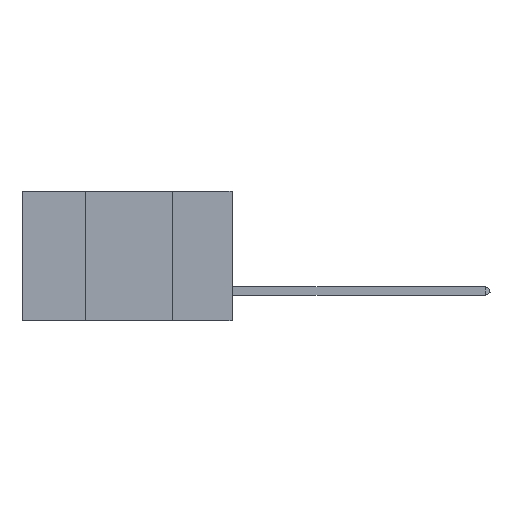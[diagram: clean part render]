
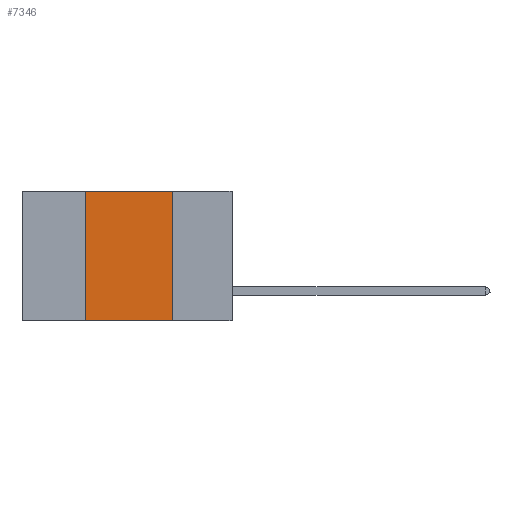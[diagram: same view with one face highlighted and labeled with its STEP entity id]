
A CAD part, left-side view. The second image highlights one B-rep face of the part: STEP entity #7346.
In plain terms, the highlighted planar face has unit normal (-1, 0, 0).
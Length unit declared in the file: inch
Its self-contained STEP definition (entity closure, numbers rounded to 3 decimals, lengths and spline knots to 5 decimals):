
#81 = CARTESIAN_POINT ( 'NONE',  ( 0., 0.6, 0. ) ) ;
#466 = CARTESIAN_POINT ( 'NONE',  ( 0., 0.17, 0. ) ) ;
#743 = EDGE_CURVE ( 'NONE', #13435, #10442, #17236, .T. ) ;
#807 = LINE ( 'NONE', #81, #6504 ) ;
#971 = CARTESIAN_POINT ( 'NONE',  ( 0., 0.6, -0.37 ) ) ;
#2218 = EDGE_LOOP ( 'NONE', ( #6266, #3308, #15476, #9253 ) ) ;
#3107 = LINE ( 'NONE', #971, #4818 ) ;
#3308 = ORIENTED_EDGE ( 'NONE', *, *, #3392, .F. ) ;
#3386 = DIRECTION ( 'NONE',  ( 0., 0., 1. ) ) ;
#3392 = EDGE_CURVE ( 'NONE', #9816, #13435, #807, .T. ) ;
#4089 = DIRECTION ( 'NONE',  ( 1., 0., 0. ) ) ;
#4458 = EDGE_CURVE ( 'NONE', #15866, #9816, #14461, .T. ) ;
#4818 = VECTOR ( 'NONE', #11678, 39.37008 ) ;
#5842 = CARTESIAN_POINT ( 'NONE',  ( 0., 0.17, -0.37 ) ) ;
#6266 = ORIENTED_EDGE ( 'NONE', *, *, #743, .F. ) ;
#6504 = VECTOR ( 'NONE', #17432, 39.37008 ) ;
#6873 = CARTESIAN_POINT ( 'NONE',  ( 0., 0.17, 0. ) ) ;
#6984 = CARTESIAN_POINT ( 'NONE',  ( 0., 0.42, -0.37 ) ) ;
#7245 = AXIS2_PLACEMENT_3D ( 'NONE', #13342, #4089, #10845 ) ;
#7313 = CARTESIAN_POINT ( 'NONE',  ( 0., 0.42, 0. ) ) ;
#7346 = ADVANCED_FACE ( 'NONE', ( #11368 ), #10675, .F. ) ;
#8486 = DIRECTION ( 'NONE',  ( 0., 0., -1. ) ) ;
#9253 = ORIENTED_EDGE ( 'NONE', *, *, #16838, .T. ) ;
#9453 = CARTESIAN_POINT ( 'NONE',  ( 0., 0.42, 0. ) ) ;
#9816 = VERTEX_POINT ( 'NONE', #9453 ) ;
#10442 = VERTEX_POINT ( 'NONE', #5842 ) ;
#10629 = VECTOR ( 'NONE', #3386, 39.37008 ) ;
#10675 = PLANE ( 'NONE',  #7245 ) ;
#10845 = DIRECTION ( 'NONE',  ( 0., 0., -1. ) ) ;
#11368 = FACE_OUTER_BOUND ( 'NONE', #2218, .T. ) ;
#11678 = DIRECTION ( 'NONE',  ( 0., -1., 0. ) ) ;
#13342 = CARTESIAN_POINT ( 'NONE',  ( 0., 0.6, 0. ) ) ;
#13435 = VERTEX_POINT ( 'NONE', #6873 ) ;
#14043 = VECTOR ( 'NONE', #8486, 39.37008 ) ;
#14461 = LINE ( 'NONE', #7313, #10629 ) ;
#15476 = ORIENTED_EDGE ( 'NONE', *, *, #4458, .F. ) ;
#15866 = VERTEX_POINT ( 'NONE', #6984 ) ;
#16838 = EDGE_CURVE ( 'NONE', #15866, #10442, #3107, .T. ) ;
#17236 = LINE ( 'NONE', #466, #14043 ) ;
#17432 = DIRECTION ( 'NONE',  ( 0., -1., 0. ) ) ;
